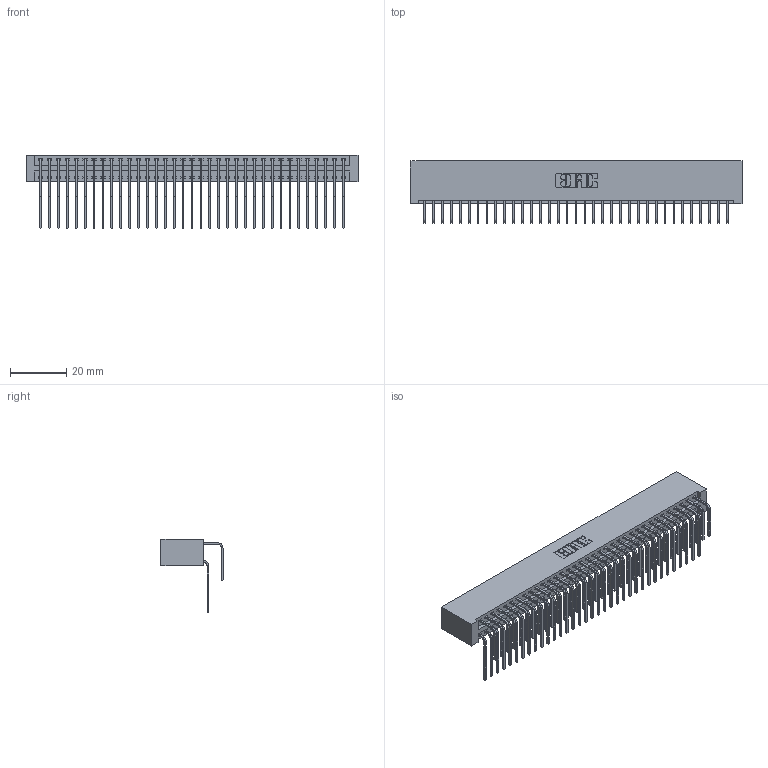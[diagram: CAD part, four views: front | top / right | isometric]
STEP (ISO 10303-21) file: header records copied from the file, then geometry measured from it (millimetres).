
FILE_DESCRIPTION (( 'STEP AP203' ), '1' );
FILE_NAME ('346-070-558-201.STEP', '2022-05-24T22:14:42', ( '' ), ( '' ), 'SwSTEP 2.0', 'SolidWorks 2020', '' );
FILE_SCHEMA (( 'CONFIG_CONTROL_DESIGN' ));
Length unit declared in the file: inch
Products named in the file (4): 345-292-001_558 559 Tail - 1; 346 Part_No Mounting Lugs; 346-070-558-201; 345-292-001_558 Tail - 2
Assembly tree (71 placements, depth 2):
  346-070-558-201
    346 Part_No Mounting Lugs
    345-292-001_558 559 Tail - 1  x35
    345-292-001_558 Tail - 2  x35
Bounding box: 118.36 x 22.16 x 26.16 mm (x, y, z)
Volume: 12464.7 mm3; surface area: 19123.9 mm2
Topology: 71 solids, 71 shells, 3894 faces, 11575 edges, 7622 vertices
Faces by surface type: plane 2662, cylinder 1232
Entity records: 25291 total; most frequent: CARTESIAN_POINT 4227, ORIENTED_EDGE 4110, DIRECTION 3743, EDGE_CURVE 2055, LINE 1751, VECTOR 1751, VERTEX_POINT 1366, AXIS2_PLACEMENT_3D 996
